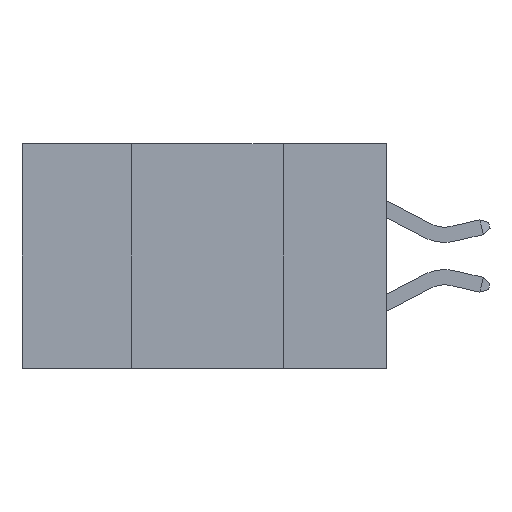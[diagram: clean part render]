
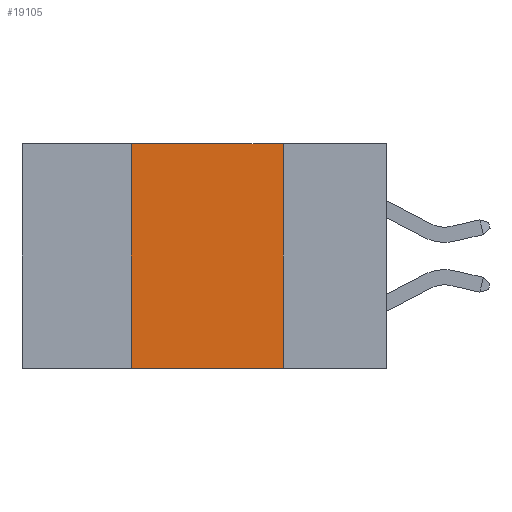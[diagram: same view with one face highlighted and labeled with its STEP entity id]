
A CAD part, left-side view. The second image highlights one B-rep face of the part: STEP entity #19105.
In plain terms, the highlighted planar face has unit normal (-1, 0, 0).
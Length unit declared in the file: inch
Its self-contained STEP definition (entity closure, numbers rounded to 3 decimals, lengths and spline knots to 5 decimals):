
#565 = PLANE ( 'NONE',  #2624 ) ;
#1454 = CARTESIAN_POINT ( 'NONE',  ( 0., 0.42, 0. ) ) ;
#1743 = DIRECTION ( 'NONE',  ( 0., -1., 0. ) ) ;
#2083 = DIRECTION ( 'NONE',  ( 0., 0., -1. ) ) ;
#2245 = CARTESIAN_POINT ( 'NONE',  ( 0., 0.6, 0. ) ) ;
#2446 = VERTEX_POINT ( 'NONE', #17857 ) ;
#2563 = VECTOR ( 'NONE', #4937, 39.37008 ) ;
#2622 = VERTEX_POINT ( 'NONE', #14051 ) ;
#2624 = AXIS2_PLACEMENT_3D ( 'NONE', #16954, #11115, #2083 ) ;
#3136 = CARTESIAN_POINT ( 'NONE',  ( 0., 0.6, -0.37 ) ) ;
#3420 = CARTESIAN_POINT ( 'NONE',  ( 0., 0.17, 0. ) ) ;
#4657 = VERTEX_POINT ( 'NONE', #5429 ) ;
#4937 = DIRECTION ( 'NONE',  ( 0., 0., -1. ) ) ;
#5429 = CARTESIAN_POINT ( 'NONE',  ( 0., 0.42, -0.37 ) ) ;
#5678 = VECTOR ( 'NONE', #1743, 39.37008 ) ;
#8341 = DIRECTION ( 'NONE',  ( 0., -1., 0. ) ) ;
#9725 = ORIENTED_EDGE ( 'NONE', *, *, #19067, .F. ) ;
#10488 = DIRECTION ( 'NONE',  ( 0., 0., 1. ) ) ;
#10622 = LINE ( 'NONE', #1454, #14101 ) ;
#11115 = DIRECTION ( 'NONE',  ( 1., 0., 0. ) ) ;
#11473 = VECTOR ( 'NONE', #8341, 39.37008 ) ;
#13916 = EDGE_LOOP ( 'NONE', ( #9725, #14158, #15092, #15110 ) ) ;
#14051 = CARTESIAN_POINT ( 'NONE',  ( 0., 0.17, -0.37 ) ) ;
#14101 = VECTOR ( 'NONE', #10488, 39.37008 ) ;
#14158 = ORIENTED_EDGE ( 'NONE', *, *, #14463, .F. ) ;
#14463 = EDGE_CURVE ( 'NONE', #14937, #2446, #19242, .T. ) ;
#14923 = LINE ( 'NONE', #3420, #2563 ) ;
#14937 = VERTEX_POINT ( 'NONE', #19183 ) ;
#15092 = ORIENTED_EDGE ( 'NONE', *, *, #18114, .F. ) ;
#15110 = ORIENTED_EDGE ( 'NONE', *, *, #17140, .T. ) ;
#16954 = CARTESIAN_POINT ( 'NONE',  ( 0., 0.6, 0. ) ) ;
#17140 = EDGE_CURVE ( 'NONE', #4657, #2622, #17543, .T. ) ;
#17543 = LINE ( 'NONE', #3136, #5678 ) ;
#17857 = CARTESIAN_POINT ( 'NONE',  ( 0., 0.17, 0. ) ) ;
#17984 = FACE_OUTER_BOUND ( 'NONE', #13916, .T. ) ;
#18114 = EDGE_CURVE ( 'NONE', #4657, #14937, #10622, .T. ) ;
#19067 = EDGE_CURVE ( 'NONE', #2446, #2622, #14923, .T. ) ;
#19105 = ADVANCED_FACE ( 'NONE', ( #17984 ), #565, .F. ) ;
#19183 = CARTESIAN_POINT ( 'NONE',  ( 0., 0.42, 0. ) ) ;
#19242 = LINE ( 'NONE', #2245, #11473 ) ;
